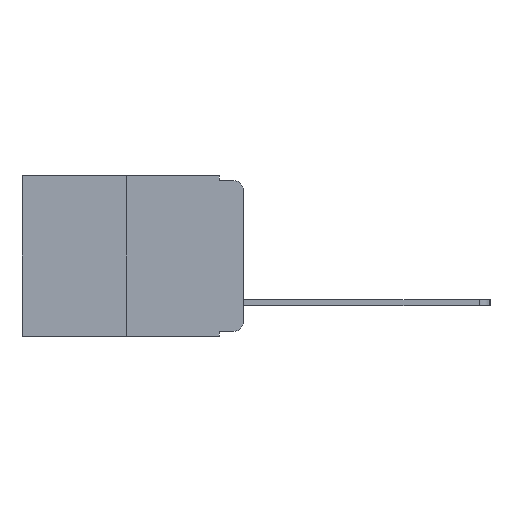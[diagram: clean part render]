
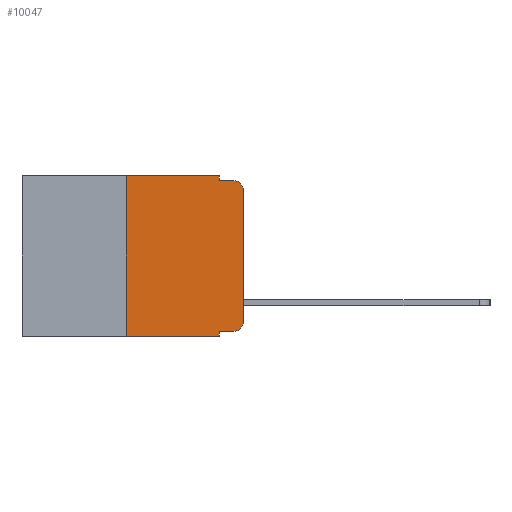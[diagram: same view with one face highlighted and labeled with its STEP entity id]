
A CAD part, left-side view. The second image highlights one B-rep face of the part: STEP entity #10047.
In plain terms, the highlighted planar face has unit normal (-1, 0, 0).
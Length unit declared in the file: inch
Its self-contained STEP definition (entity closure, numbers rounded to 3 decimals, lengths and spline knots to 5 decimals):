
#161 = DIRECTION ( 'NONE',  ( -1., 0., 0. ) ) ;
#411 = CARTESIAN_POINT ( 'NONE',  ( 0., 0.473, 0. ) ) ;
#553 = DIRECTION ( 'NONE',  ( 0., 0., -1. ) ) ;
#765 = CARTESIAN_POINT ( 'NONE',  ( 0., 0., -0.03 ) ) ;
#800 = EDGE_CURVE ( 'NONE', #17646, #1765, #2509, .T. ) ;
#1309 = DIRECTION ( 'NONE',  ( 0., -1., 0. ) ) ;
#1582 = VERTEX_POINT ( 'NONE', #1965 ) ;
#1765 = VERTEX_POINT ( 'NONE', #13104 ) ;
#1814 = VECTOR ( 'NONE', #3584, 39.37008 ) ;
#1907 = EDGE_CURVE ( 'NONE', #1765, #8119, #1968, .T. ) ;
#1965 = CARTESIAN_POINT ( 'NONE',  ( 0., 0.051, -0.333 ) ) ;
#1968 = LINE ( 'NONE', #6043, #4667 ) ;
#2509 = LINE ( 'NONE', #3261, #10255 ) ;
#2564 = ORIENTED_EDGE ( 'NONE', *, *, #8188, .T. ) ;
#2932 = VECTOR ( 'NONE', #16078, 39.37008 ) ;
#2978 = CARTESIAN_POINT ( 'NONE',  ( 0., 0.051, -0.343 ) ) ;
#3117 = VERTEX_POINT ( 'NONE', #16946 ) ;
#3261 = CARTESIAN_POINT ( 'NONE',  ( 0., 0.051, 0. ) ) ;
#3317 = ORIENTED_EDGE ( 'NONE', *, *, #13100, .T. ) ;
#3584 = DIRECTION ( 'NONE',  ( 0., -1., 0. ) ) ;
#3704 = VERTEX_POINT ( 'NONE', #14944 ) ;
#3935 = LINE ( 'NONE', #4762, #11153 ) ;
#4417 = ORIENTED_EDGE ( 'NONE', *, *, #9231, .F. ) ;
#4615 = AXIS2_PLACEMENT_3D ( 'NONE', #9579, #161, #11090 ) ;
#4667 = VECTOR ( 'NONE', #1309, 39.37008 ) ;
#4762 = CARTESIAN_POINT ( 'NONE',  ( 0., 0.473, -0.343 ) ) ;
#4888 = CARTESIAN_POINT ( 'NONE',  ( 0., 0.25, 0. ) ) ;
#5249 = VERTEX_POINT ( 'NONE', #765 ) ;
#5284 = DIRECTION ( 'NONE',  ( -1., 0., 0. ) ) ;
#5699 = ORIENTED_EDGE ( 'NONE', *, *, #17706, .T. ) ;
#6043 = CARTESIAN_POINT ( 'NONE',  ( 0., 0.051, -0.01 ) ) ;
#6184 = DIRECTION ( 'NONE',  ( 0., 0., -1. ) ) ;
#6625 = VECTOR ( 'NONE', #16652, 39.37008 ) ;
#6786 = CARTESIAN_POINT ( 'NONE',  ( 0., 0.473, 0. ) ) ;
#6801 = CARTESIAN_POINT ( 'NONE',  ( 0., 0.051, -0.333 ) ) ;
#7188 = VERTEX_POINT ( 'NONE', #15253 ) ;
#7842 = LINE ( 'NONE', #6801, #11359 ) ;
#8119 = VERTEX_POINT ( 'NONE', #9652 ) ;
#8188 = EDGE_CURVE ( 'NONE', #5249, #8119, #13080, .T. ) ;
#8307 = DIRECTION ( 'NONE',  ( 0., -1., 0. ) ) ;
#8359 = AXIS2_PLACEMENT_3D ( 'NONE', #411, #9901, #553 ) ;
#9224 = CARTESIAN_POINT ( 'NONE',  ( 0., 0.051, 0. ) ) ;
#9231 = EDGE_CURVE ( 'NONE', #3704, #17646, #12980, .T. ) ;
#9579 = CARTESIAN_POINT ( 'NONE',  ( 0., 0.02, -0.313 ) ) ;
#9652 = CARTESIAN_POINT ( 'NONE',  ( 0., 0.02, -0.01 ) ) ;
#9901 = DIRECTION ( 'NONE',  ( 1., 0., 0. ) ) ;
#10047 = ADVANCED_FACE ( 'NONE', ( #12283 ), #18436, .F. ) ;
#10255 = VECTOR ( 'NONE', #6184, 39.37008 ) ;
#10624 = LINE ( 'NONE', #4888, #6625 ) ;
#10673 = CARTESIAN_POINT ( 'NONE',  ( 0., 0., 0. ) ) ;
#10871 = LINE ( 'NONE', #10673, #17938 ) ;
#11090 = DIRECTION ( 'NONE',  ( 0., 0., -1. ) ) ;
#11153 = VECTOR ( 'NONE', #17961, 39.37008 ) ;
#11359 = VECTOR ( 'NONE', #8307, 39.37008 ) ;
#11370 = ORIENTED_EDGE ( 'NONE', *, *, #19134, .F. ) ;
#12112 = DIRECTION ( 'NONE',  ( 0., 0., 1. ) ) ;
#12283 = FACE_OUTER_BOUND ( 'NONE', #16149, .T. ) ;
#12479 = ORIENTED_EDGE ( 'NONE', *, *, #12505, .T. ) ;
#12505 = EDGE_CURVE ( 'NONE', #3117, #16383, #18840, .T. ) ;
#12980 = LINE ( 'NONE', #6786, #1814 ) ;
#13080 = CIRCLE ( 'NONE', #18561, 0.02 ) ;
#13100 = EDGE_CURVE ( 'NONE', #16383, #5249, #10871, .T. ) ;
#13104 = CARTESIAN_POINT ( 'NONE',  ( 0., 0.051, -0.01 ) ) ;
#14154 = CARTESIAN_POINT ( 'NONE',  ( 0., 0.02, -0.03 ) ) ;
#14329 = ORIENTED_EDGE ( 'NONE', *, *, #1907, .F. ) ;
#14650 = ORIENTED_EDGE ( 'NONE', *, *, #17222, .T. ) ;
#14660 = CARTESIAN_POINT ( 'NONE',  ( 0., 0.051, 0. ) ) ;
#14866 = LINE ( 'NONE', #14660, #2932 ) ;
#14944 = CARTESIAN_POINT ( 'NONE',  ( 0., 0.25, 0. ) ) ;
#15253 = CARTESIAN_POINT ( 'NONE',  ( 0., 0.25, -0.343 ) ) ;
#15293 = ORIENTED_EDGE ( 'NONE', *, *, #800, .F. ) ;
#15568 = DIRECTION ( 'NONE',  ( 0., 0., -1. ) ) ;
#16078 = DIRECTION ( 'NONE',  ( 0., 0., -1. ) ) ;
#16140 = CARTESIAN_POINT ( 'NONE',  ( 0., 0., -0.313 ) ) ;
#16149 = EDGE_LOOP ( 'NONE', ( #3317, #2564, #14329, #15293, #4417, #11370, #5699, #16672, #14650, #12479 ) ) ;
#16383 = VERTEX_POINT ( 'NONE', #16140 ) ;
#16652 = DIRECTION ( 'NONE',  ( 0., 0., 1. ) ) ;
#16672 = ORIENTED_EDGE ( 'NONE', *, *, #18183, .F. ) ;
#16946 = CARTESIAN_POINT ( 'NONE',  ( 0., 0.02, -0.333 ) ) ;
#17222 = EDGE_CURVE ( 'NONE', #1582, #3117, #7842, .T. ) ;
#17621 = VERTEX_POINT ( 'NONE', #2978 ) ;
#17646 = VERTEX_POINT ( 'NONE', #9224 ) ;
#17706 = EDGE_CURVE ( 'NONE', #7188, #17621, #3935, .T. ) ;
#17938 = VECTOR ( 'NONE', #12112, 39.37008 ) ;
#17961 = DIRECTION ( 'NONE',  ( 0., -1., 0. ) ) ;
#18183 = EDGE_CURVE ( 'NONE', #1582, #17621, #14866, .T. ) ;
#18436 = PLANE ( 'NONE',  #8359 ) ;
#18561 = AXIS2_PLACEMENT_3D ( 'NONE', #14154, #5284, #15568 ) ;
#18840 = CIRCLE ( 'NONE', #4615, 0.02 ) ;
#19134 = EDGE_CURVE ( 'NONE', #7188, #3704, #10624, .T. ) ;
